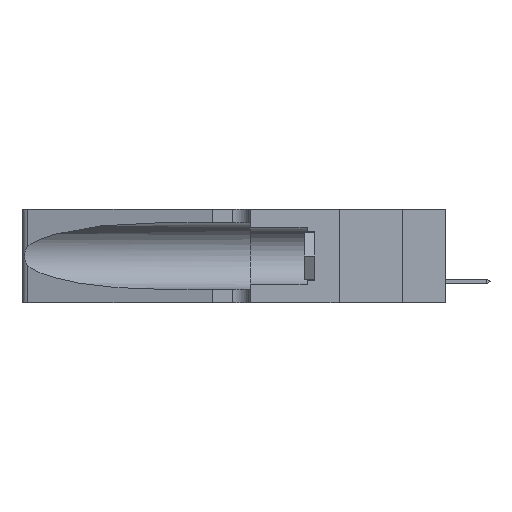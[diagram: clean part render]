
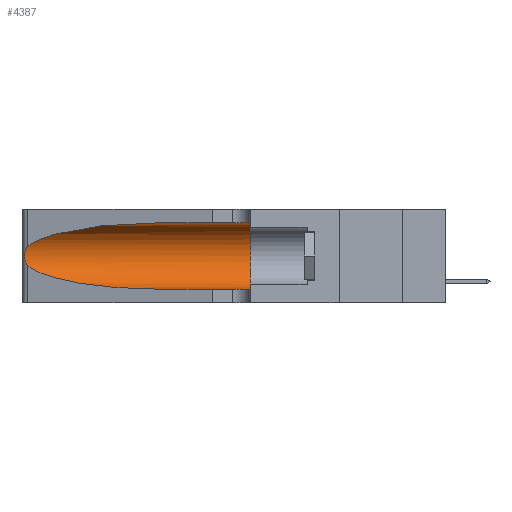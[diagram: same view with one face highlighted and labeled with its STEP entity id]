
A CAD part, left-side view. The second image highlights one B-rep face of the part: STEP entity #4387.
In plain terms, the highlighted cylindrical face has radius 3.308 mm (diameter 6.617 mm), a partial arc.
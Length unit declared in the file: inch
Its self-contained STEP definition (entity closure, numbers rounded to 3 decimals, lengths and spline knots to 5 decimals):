
#33 = VERTEX_POINT ( 'NONE', #5650 ) ;
#800 = ORIENTED_EDGE ( 'NONE', *, *, #26265, .F. ) ;
#1849 = CARTESIAN_POINT ( 'NONE',  ( 0.1305, 1.61858, 0.185 ) ) ;
#2014 = DIRECTION ( 'NONE',  ( 0., 1., 0. ) ) ;
#2173 = CARTESIAN_POINT ( 'NONE',  ( 0.25487, 1.22718, 0.22369 ) ) ;
#2964 = LINE ( 'NONE', #11907, #25146 ) ;
#2967 = CARTESIAN_POINT ( 'NONE',  ( 0.1305, 0.72297, 0.31525 ) ) ;
#4387 = ADVANCED_FACE ( 'NONE', ( #22653 ), #18971, .F. ) ;
#5062 = AXIS2_PLACEMENT_3D ( 'NONE', #27675, #2014, #10384 ) ;
#5240 = CARTESIAN_POINT ( 'NONE',  ( 0.25487, 1.22718, 0.22369 ) ) ;
#5650 = CARTESIAN_POINT ( 'NONE',  ( 0.1305, 0.35, 0.31525 ) ) ;
#6258 = CARTESIAN_POINT ( 'NONE',  ( 0.26017, 1.23833, 0.17102 ) ) ;
#6349 = CARTESIAN_POINT ( 'NONE',  ( 0.25639, 1.23184, 0.21858 ) ) ;
#6536 = CARTESIAN_POINT ( 'NONE',  ( 0.25487, 1.22718, 0.22369 ) ) ;
#7895 = VERTEX_POINT ( 'NONE', #18100 ) ;
#8239 = VERTEX_POINT ( 'NONE', #2173 ) ;
#8271 = ORIENTED_EDGE ( 'NONE', *, *, #13683, .T. ) ;
#10384 = DIRECTION ( 'NONE',  ( 0., 0., 1. ) ) ;
#10475 = CARTESIAN_POINT ( 'NONE',  ( 0.25787, 1.23484, 0.2124 ) ) ;
#10560 = CARTESIAN_POINT ( 'NONE',  ( 0.25789, 1.23486, 0.15765 ) ) ;
#10748 = CARTESIAN_POINT ( 'NONE',  ( 0.25555, 1.22994, 0.2215 ) ) ;
#10806 = EDGE_CURVE ( 'NONE', #33, #19549, #21240, .T. ) ;
#11887 = EDGE_CURVE ( 'NONE', #7895, #8239, #18192, .T. ) ;
#11907 = CARTESIAN_POINT ( 'NONE',  ( 0.1305, 1.61858, 0.31525 ) ) ;
#12001 = DIRECTION ( 'NONE',  ( 0., -1., 0. ) ) ;
#12531 = CARTESIAN_POINT ( 'NONE',  ( 0.25856, 1.23593, 0.16098 ) ) ;
#13632 = ORIENTED_EDGE ( 'NONE', *, *, #23617, .T. ) ;
#13663 = CARTESIAN_POINT ( 'NONE',  ( 0.1305, 0.72297, 0.05475 ) ) ;
#13683 = EDGE_CURVE ( 'NONE', #20832, #16757, #14558, .T. ) ;
#13986 = CARTESIAN_POINT ( 'NONE',  ( 0.1305, 0.72297, 0.05475 ) ) ;
#14351 = LINE ( 'NONE', #25547, #23413 ) ;
#14558 =( BOUNDED_CURVE ( )  B_SPLINE_CURVE ( 3, ( #26639, #18181, #20320, #13663 ),
 .UNSPECIFIED., .F., .F. ) 
 B_SPLINE_CURVE_WITH_KNOTS ( ( 4, 4 ),
 ( 3.44316, 4.71239 ),
 .UNSPECIFIED. ) 
 CURVE ( )  GEOMETRIC_REPRESENTATION_ITEM ( )  RATIONAL_B_SPLINE_CURVE ( ( 1., 0.87, 0.87, 1. ) ) 
 REPRESENTATION_ITEM ( '' )  );
#15087 = CARTESIAN_POINT ( 'NONE',  ( 0.25854, 1.2359, 0.20912 ) ) ;
#16757 = VERTEX_POINT ( 'NONE', #13986 ) ;
#16903 = DIRECTION ( 'NONE',  ( 0., -1., 0. ) ) ;
#16974 = CARTESIAN_POINT ( 'NONE',  ( 0.25639, 1.23186, 0.15144 ) ) ;
#17381 = CARTESIAN_POINT ( 'NONE',  ( 0.25487, 1.22718, 0.14631 ) ) ;
#18100 = CARTESIAN_POINT ( 'NONE',  ( 0.1305, 0.72297, 0.31525 ) ) ;
#18181 = CARTESIAN_POINT ( 'NONE',  ( 0.2373, 1.15595, 0.08982 ) ) ;
#18192 =( BOUNDED_CURVE ( )  B_SPLINE_CURVE ( 3, ( #2967, #22151, #22409, #5240 ),
 .UNSPECIFIED., .F., .F. ) 
 B_SPLINE_CURVE_WITH_KNOTS ( ( 4, 4 ),
 ( 1.5708, 2.84003 ),
 .UNSPECIFIED. ) 
 CURVE ( )  GEOMETRIC_REPRESENTATION_ITEM ( )  RATIONAL_B_SPLINE_CURVE ( ( 1., 0.87, 0.87, 1. ) ) 
 REPRESENTATION_ITEM ( '' )  );
#18506 = ORIENTED_EDGE ( 'NONE', *, *, #10806, .F. ) ;
#18971 = CYLINDRICAL_SURFACE ( 'NONE', #22925, 0.13025 ) ;
#19126 = CARTESIAN_POINT ( 'NONE',  ( 0.25487, 1.22718, 0.14631 ) ) ;
#19211 = CARTESIAN_POINT ( 'NONE',  ( 0.25555, 1.22993, 0.14849 ) ) ;
#19243 = DIRECTION ( 'NONE',  ( 0., -1., 0. ) ) ;
#19549 = VERTEX_POINT ( 'NONE', #25702 ) ;
#20320 = CARTESIAN_POINT ( 'NONE',  ( 0.18966, 0.96281, 0.05475 ) ) ;
#20832 = VERTEX_POINT ( 'NONE', #17381 ) ;
#20977 = EDGE_LOOP ( 'NONE', ( #26894, #22805, #8271, #13632, #18506, #800 ) ) ;
#21240 = CIRCLE ( 'NONE', #5062, 0.13025 ) ;
#22151 = CARTESIAN_POINT ( 'NONE',  ( 0.18966, 0.96281, 0.31525 ) ) ;
#22279 = EDGE_CURVE ( 'NONE', #8239, #20832, #26105, .T. ) ;
#22409 = CARTESIAN_POINT ( 'NONE',  ( 0.2373, 1.15595, 0.28018 ) ) ;
#22653 = FACE_OUTER_BOUND ( 'NONE', #20977, .T. ) ;
#22805 = ORIENTED_EDGE ( 'NONE', *, *, #22279, .T. ) ;
#22925 = AXIS2_PLACEMENT_3D ( 'NONE', #1849, #16903, #27323 ) ;
#23413 = VECTOR ( 'NONE', #19243, 39.37008 ) ;
#23617 = EDGE_CURVE ( 'NONE', #16757, #19549, #14351, .T. ) ;
#23704 = CARTESIAN_POINT ( 'NONE',  ( 0.26075, 1.23896, 0.178 ) ) ;
#25146 = VECTOR ( 'NONE', #12001, 39.37008 ) ;
#25547 = CARTESIAN_POINT ( 'NONE',  ( 0.1305, 1.61858, 0.05475 ) ) ;
#25697 = CARTESIAN_POINT ( 'NONE',  ( 0.26075, 1.23896, 0.19203 ) ) ;
#25702 = CARTESIAN_POINT ( 'NONE',  ( 0.1305, 0.35, 0.05475 ) ) ;
#26105 = B_SPLINE_CURVE_WITH_KNOTS ( 'NONE', 3,
 ( #6536, #10748, #6349, #10475, #15087, #27857, #25697, #23704, #6258, #12531, #10560, #16974, #19211, #19126 ),
 .UNSPECIFIED., .F., .F.,
 ( 4, 2, 2, 2, 2, 2, 4 ),
 ( 0., 0.00027, 0.00053, 0.00107, 0.0016, 0.00187, 0.00214 ),
 .UNSPECIFIED. ) ;
#26265 = EDGE_CURVE ( 'NONE', #7895, #33, #2964, .T. ) ;
#26639 = CARTESIAN_POINT ( 'NONE',  ( 0.25487, 1.22718, 0.14631 ) ) ;
#26894 = ORIENTED_EDGE ( 'NONE', *, *, #11887, .T. ) ;
#27323 = DIRECTION ( 'NONE',  ( 0., 0., -1. ) ) ;
#27675 = CARTESIAN_POINT ( 'NONE',  ( 0.1305, 0.35, 0.185 ) ) ;
#27857 = CARTESIAN_POINT ( 'NONE',  ( 0.26018, 1.23835, 0.19895 ) ) ;
